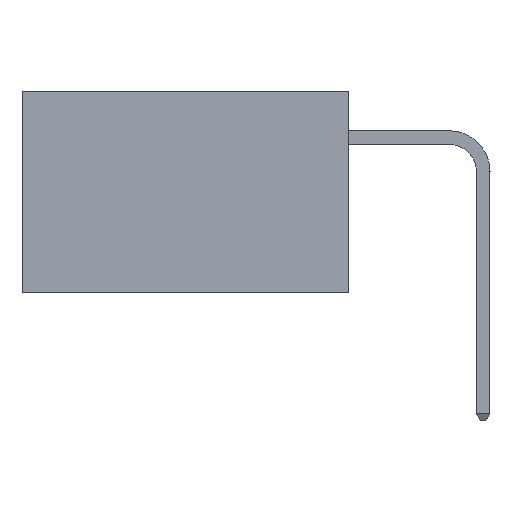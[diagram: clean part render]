
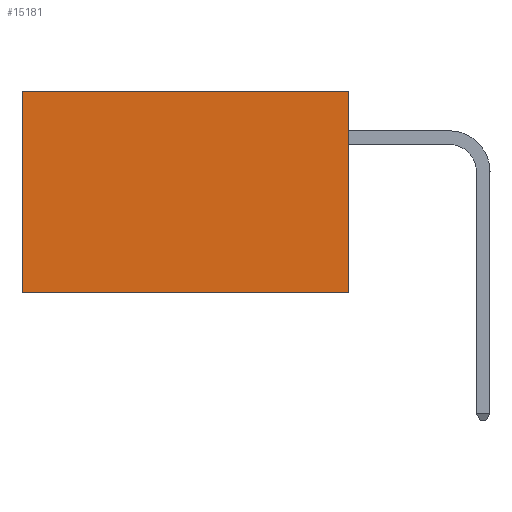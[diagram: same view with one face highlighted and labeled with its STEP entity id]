
A CAD part, left-side view. The second image highlights one B-rep face of the part: STEP entity #15181.
In plain terms, the highlighted planar face has unit normal (-1, 0, 0).
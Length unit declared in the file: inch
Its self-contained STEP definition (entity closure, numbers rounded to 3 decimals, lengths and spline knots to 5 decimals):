
#2232 = FACE_OUTER_BOUND ( 'NONE', #4367, .T. ) ;
#3117 = CARTESIAN_POINT ( 'NONE',  ( 0.2875, 0., 0. ) ) ;
#3901 = CARTESIAN_POINT ( 'NONE',  ( 0.2875, 0.6, 0. ) ) ;
#4367 = EDGE_LOOP ( 'NONE', ( #5409, #9172, #29230, #9447 ) ) ;
#5146 = VERTEX_POINT ( 'NONE', #3901 ) ;
#5409 = ORIENTED_EDGE ( 'NONE', *, *, #10099, .T. ) ;
#5890 = LINE ( 'NONE', #16620, #18713 ) ;
#6386 = LINE ( 'NONE', #21703, #18504 ) ;
#7241 = LINE ( 'NONE', #23928, #18654 ) ;
#7369 = VERTEX_POINT ( 'NONE', #23397 ) ;
#7566 = DIRECTION ( 'NONE',  ( 0., 1., 0. ) ) ;
#8031 = EDGE_CURVE ( 'NONE', #10020, #5146, #5890, .T. ) ;
#9172 = ORIENTED_EDGE ( 'NONE', *, *, #16084, .F. ) ;
#9447 = ORIENTED_EDGE ( 'NONE', *, *, #8031, .T. ) ;
#10020 = VERTEX_POINT ( 'NONE', #3117 ) ;
#10099 = EDGE_CURVE ( 'NONE', #5146, #7369, #6386, .T. ) ;
#12595 = DIRECTION ( 'NONE',  ( 0., 1., 0. ) ) ;
#13735 = CARTESIAN_POINT ( 'NONE',  ( 0.2875, 0., 0. ) ) ;
#15181 = ADVANCED_FACE ( 'NONE', ( #2232 ), #27266, .F. ) ;
#16034 = DIRECTION ( 'NONE',  ( 0., 0., -1. ) ) ;
#16084 = EDGE_CURVE ( 'NONE', #23820, #7369, #7241, .T. ) ;
#16620 = CARTESIAN_POINT ( 'NONE',  ( 0.2875, 0., 0. ) ) ;
#18504 = VECTOR ( 'NONE', #23949, 39.37008 ) ;
#18654 = VECTOR ( 'NONE', #12595, 39.37008 ) ;
#18713 = VECTOR ( 'NONE', #7566, 39.37008 ) ;
#19697 = CARTESIAN_POINT ( 'NONE',  ( 0.2875, 0., -0.37 ) ) ;
#21003 = DIRECTION ( 'NONE',  ( 0., 0., -1. ) ) ;
#21070 = VECTOR ( 'NONE', #21003, 39.37008 ) ;
#21703 = CARTESIAN_POINT ( 'NONE',  ( 0.2875, 0.6, 0. ) ) ;
#23397 = CARTESIAN_POINT ( 'NONE',  ( 0.2875, 0.6, -0.37 ) ) ;
#23537 = EDGE_CURVE ( 'NONE', #10020, #23820, #27002, .T. ) ;
#23820 = VERTEX_POINT ( 'NONE', #19697 ) ;
#23928 = CARTESIAN_POINT ( 'NONE',  ( 0.2875, 0., -0.37 ) ) ;
#23949 = DIRECTION ( 'NONE',  ( 0., 0., -1. ) ) ;
#25483 = CARTESIAN_POINT ( 'NONE',  ( 0.2875, 0., 0. ) ) ;
#27002 = LINE ( 'NONE', #25483, #21070 ) ;
#27266 = PLANE ( 'NONE',  #28356 ) ;
#28356 = AXIS2_PLACEMENT_3D ( 'NONE', #13735, #29516, #16034 ) ;
#29230 = ORIENTED_EDGE ( 'NONE', *, *, #23537, .F. ) ;
#29516 = DIRECTION ( 'NONE',  ( 1., 0., 0. ) ) ;
